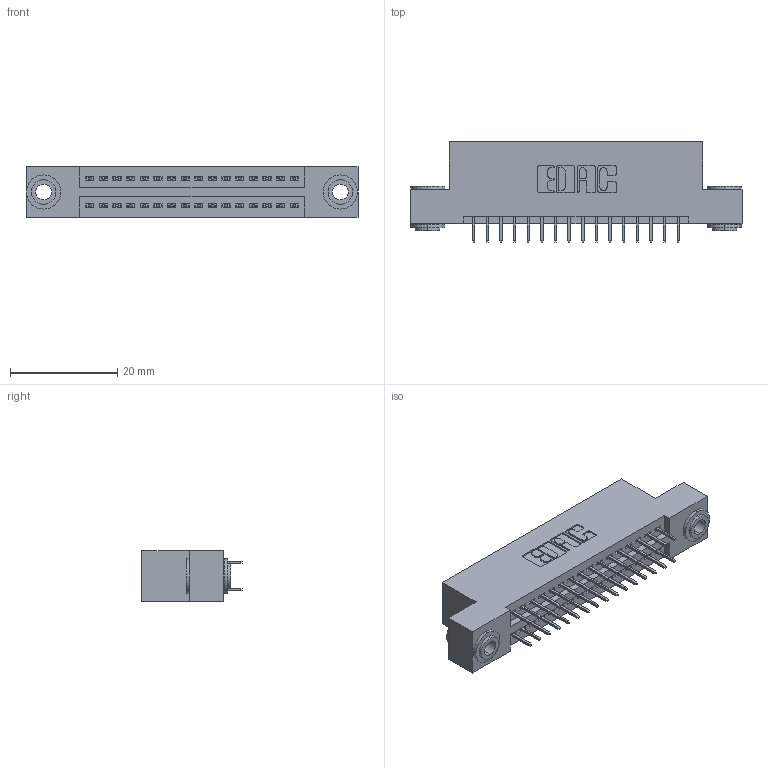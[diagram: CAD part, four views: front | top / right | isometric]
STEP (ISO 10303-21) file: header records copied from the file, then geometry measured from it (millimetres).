
FILE_DESCRIPTION (( 'STEP AP203' ), '1' );
FILE_NAME ('845-032-525-203.STEP', '2020-09-23T01:01:08', ( '' ), ( '' ), 'SwSTEP 2.0', 'SolidWorks 2020', '' );
FILE_SCHEMA (( 'CONFIG_CONTROL_DESIGN' ));
Length unit declared in the file: inch
Products named in the file (4): 345-292-001_345-293-125; 845 Part_Flush Mounting Lugs - 0.156 Dia-TH; 345-250-002_345-250-002-102; 845-032-525-203
Assembly tree (35 placements, depth 2):
  845-032-525-203
    845 Part_Flush Mounting Lugs - 0.156 Dia-TH
    345-292-001_345-293-125  x32
    345-250-002_345-250-002-102  x2
Bounding box: 61.85 x 18.72 x 9.4 mm (x, y, z)
Volume: 5733.5 mm3; surface area: 8017.6 mm2
Topology: 35 solids, 35 shells, 1892 faces, 5313 edges, 3410 vertices
Faces by surface type: plane 1338, cylinder 546, cone 8
Entity records: 16778 total; most frequent: CARTESIAN_POINT 2811, ORIENTED_EDGE 2738, DIRECTION 2543, EDGE_CURVE 1369, LINE 1153, VECTOR 1153, VERTEX_POINT 906, AXIS2_PLACEMENT_3D 695
